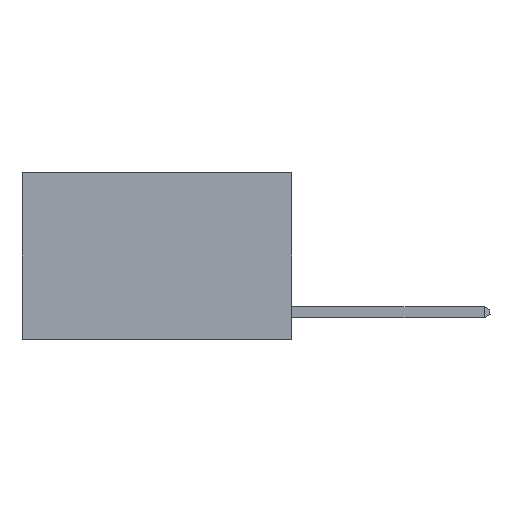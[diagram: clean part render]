
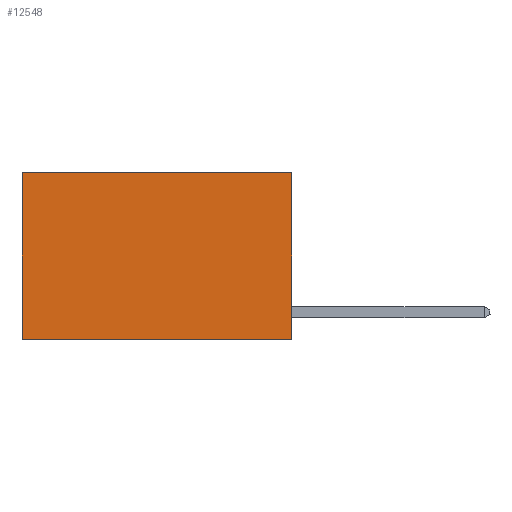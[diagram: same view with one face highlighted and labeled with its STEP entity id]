
A CAD part, left-side view. The second image highlights one B-rep face of the part: STEP entity #12548.
In plain terms, the highlighted planar face has unit normal (-1, 0, 0).
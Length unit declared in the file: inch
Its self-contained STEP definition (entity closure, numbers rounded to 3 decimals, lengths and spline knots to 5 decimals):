
#20 = EDGE_CURVE ( 'NONE', #14142, #5310, #16894, .T. ) ;
#1707 = DIRECTION ( 'NONE',  ( 0., 0., -1. ) ) ;
#2979 = DIRECTION ( 'NONE',  ( 0., 1., 0. ) ) ;
#3724 = CARTESIAN_POINT ( 'NONE',  ( 0.2625, 0., 0. ) ) ;
#3822 = DIRECTION ( 'NONE',  ( 0., 1., 0. ) ) ;
#4169 = VERTEX_POINT ( 'NONE', #17480 ) ;
#4521 = FACE_OUTER_BOUND ( 'NONE', #4680, .T. ) ;
#4680 = EDGE_LOOP ( 'NONE', ( #15150, #7128, #12774, #13962 ) ) ;
#5310 = VERTEX_POINT ( 'NONE', #17295 ) ;
#5859 = LINE ( 'NONE', #14512, #16791 ) ;
#6227 = CARTESIAN_POINT ( 'NONE',  ( 0.2625, 0.6, 0. ) ) ;
#6617 = DIRECTION ( 'NONE',  ( 0., 0., -1. ) ) ;
#7128 = ORIENTED_EDGE ( 'NONE', *, *, #20, .F. ) ;
#9185 = CARTESIAN_POINT ( 'NONE',  ( 0.2625, 0., -0.37 ) ) ;
#9857 = EDGE_CURVE ( 'NONE', #4169, #11452, #13128, .T. ) ;
#10736 = CARTESIAN_POINT ( 'NONE',  ( 0.2625, 0., -0.37 ) ) ;
#10955 = CARTESIAN_POINT ( 'NONE',  ( 0.2625, 0., 0. ) ) ;
#11399 = AXIS2_PLACEMENT_3D ( 'NONE', #3724, #15143, #6617 ) ;
#11452 = VERTEX_POINT ( 'NONE', #18244 ) ;
#12548 = ADVANCED_FACE ( 'NONE', ( #4521 ), #13724, .F. ) ;
#12774 = ORIENTED_EDGE ( 'NONE', *, *, #12920, .F. ) ;
#12920 = EDGE_CURVE ( 'NONE', #4169, #14142, #5859, .T. ) ;
#13128 = LINE ( 'NONE', #10955, #16469 ) ;
#13724 = PLANE ( 'NONE',  #11399 ) ;
#13857 = VECTOR ( 'NONE', #14702, 39.37008 ) ;
#13962 = ORIENTED_EDGE ( 'NONE', *, *, #9857, .T. ) ;
#14142 = VERTEX_POINT ( 'NONE', #10736 ) ;
#14512 = CARTESIAN_POINT ( 'NONE',  ( 0.2625, 0., 0. ) ) ;
#14684 = EDGE_CURVE ( 'NONE', #11452, #5310, #17644, .T. ) ;
#14702 = DIRECTION ( 'NONE',  ( 0., 0., -1. ) ) ;
#15143 = DIRECTION ( 'NONE',  ( 1., 0., 0. ) ) ;
#15150 = ORIENTED_EDGE ( 'NONE', *, *, #14684, .T. ) ;
#16447 = VECTOR ( 'NONE', #2979, 39.37008 ) ;
#16469 = VECTOR ( 'NONE', #3822, 39.37008 ) ;
#16791 = VECTOR ( 'NONE', #1707, 39.37008 ) ;
#16894 = LINE ( 'NONE', #9185, #16447 ) ;
#17295 = CARTESIAN_POINT ( 'NONE',  ( 0.2625, 0.6, -0.37 ) ) ;
#17480 = CARTESIAN_POINT ( 'NONE',  ( 0.2625, 0., 0. ) ) ;
#17644 = LINE ( 'NONE', #6227, #13857 ) ;
#18244 = CARTESIAN_POINT ( 'NONE',  ( 0.2625, 0.6, 0. ) ) ;
